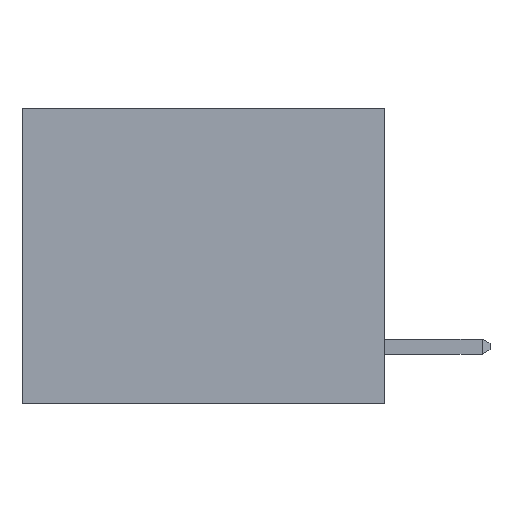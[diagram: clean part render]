
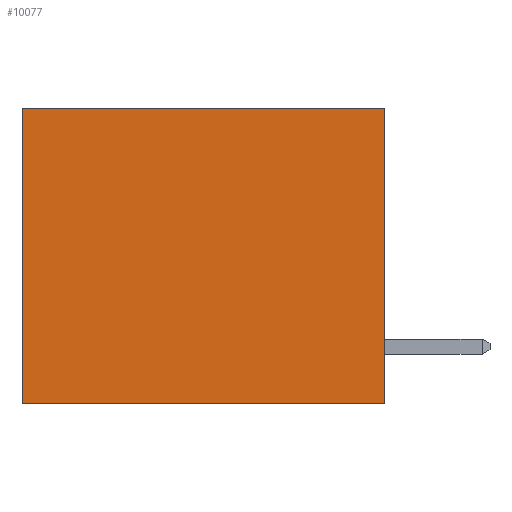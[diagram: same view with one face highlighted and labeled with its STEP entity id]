
A CAD part, left-side view. The second image highlights one B-rep face of the part: STEP entity #10077.
In plain terms, the highlighted planar face has unit normal (-1, 0, 0).
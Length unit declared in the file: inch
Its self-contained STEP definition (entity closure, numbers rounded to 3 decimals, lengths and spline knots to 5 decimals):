
#168 = EDGE_CURVE ( 'NONE', #2097, #563, #10171, .T. ) ;
#563 = VERTEX_POINT ( 'NONE', #5310 ) ;
#740 = AXIS2_PLACEMENT_3D ( 'NONE', #906, #2553, #11394 ) ;
#792 = FACE_OUTER_BOUND ( 'NONE', #6915, .T. ) ;
#906 = CARTESIAN_POINT ( 'NONE',  ( 0.3165, 0., -0.49 ) ) ;
#1322 = VECTOR ( 'NONE', #9155, 39.37008 ) ;
#1710 = PLANE ( 'NONE',  #740 ) ;
#1795 = EDGE_CURVE ( 'NONE', #2097, #2871, #10391, .T. ) ;
#2097 = VERTEX_POINT ( 'NONE', #11434 ) ;
#2191 = EDGE_CURVE ( 'NONE', #563, #3019, #3466, .T. ) ;
#2207 = CARTESIAN_POINT ( 'NONE',  ( 0.3165, 0.6, -0.49 ) ) ;
#2553 = DIRECTION ( 'NONE',  ( 1., 0., 0. ) ) ;
#2871 = VERTEX_POINT ( 'NONE', #5977 ) ;
#2998 = CARTESIAN_POINT ( 'NONE',  ( 0.3165, 0., -0.49 ) ) ;
#3019 = VERTEX_POINT ( 'NONE', #9690 ) ;
#3118 = LINE ( 'NONE', #2207, #1322 ) ;
#3466 = LINE ( 'NONE', #7083, #9679 ) ;
#3863 = DIRECTION ( 'NONE',  ( 0., 0., -1. ) ) ;
#4106 = EDGE_CURVE ( 'NONE', #2871, #3019, #3118, .T. ) ;
#4615 = ORIENTED_EDGE ( 'NONE', *, *, #1795, .T. ) ;
#4980 = VECTOR ( 'NONE', #9793, 39.37008 ) ;
#5036 = VECTOR ( 'NONE', #3863, 39.37008 ) ;
#5310 = CARTESIAN_POINT ( 'NONE',  ( 0.3165, 0., -0.49 ) ) ;
#5977 = CARTESIAN_POINT ( 'NONE',  ( 0.3165, 0.6, 0. ) ) ;
#6622 = ORIENTED_EDGE ( 'NONE', *, *, #2191, .F. ) ;
#6915 = EDGE_LOOP ( 'NONE', ( #9292, #6622, #8755, #4615 ) ) ;
#7083 = CARTESIAN_POINT ( 'NONE',  ( 0.3165, 0., -0.49 ) ) ;
#7164 = DIRECTION ( 'NONE',  ( 0., 1., 0. ) ) ;
#7301 = CARTESIAN_POINT ( 'NONE',  ( 0.3165, 0., 0. ) ) ;
#8755 = ORIENTED_EDGE ( 'NONE', *, *, #168, .F. ) ;
#9155 = DIRECTION ( 'NONE',  ( 0., 0., -1. ) ) ;
#9292 = ORIENTED_EDGE ( 'NONE', *, *, #4106, .T. ) ;
#9679 = VECTOR ( 'NONE', #7164, 39.37008 ) ;
#9690 = CARTESIAN_POINT ( 'NONE',  ( 0.3165, 0.6, -0.49 ) ) ;
#9793 = DIRECTION ( 'NONE',  ( 0., 1., 0. ) ) ;
#10077 = ADVANCED_FACE ( 'NONE', ( #792 ), #1710, .F. ) ;
#10171 = LINE ( 'NONE', #2998, #5036 ) ;
#10391 = LINE ( 'NONE', #7301, #4980 ) ;
#11394 = DIRECTION ( 'NONE',  ( 0., 0., -1. ) ) ;
#11434 = CARTESIAN_POINT ( 'NONE',  ( 0.3165, 0., 0. ) ) ;
